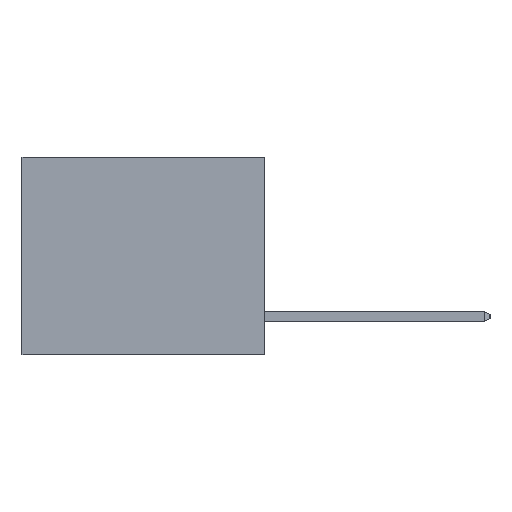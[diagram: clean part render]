
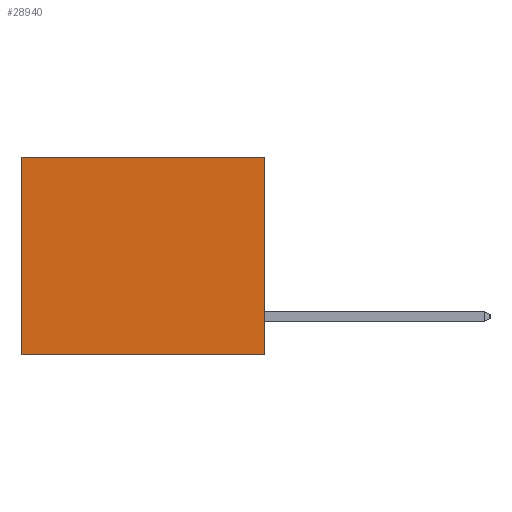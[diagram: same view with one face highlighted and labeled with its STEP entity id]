
A CAD part, left-side view. The second image highlights one B-rep face of the part: STEP entity #28940.
In plain terms, the highlighted planar face has unit normal (-1, 0, 0).
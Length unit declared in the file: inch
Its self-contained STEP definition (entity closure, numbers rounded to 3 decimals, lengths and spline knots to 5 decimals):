
#353 = LINE ( 'NONE', #3762, #6042 ) ;
#700 = CARTESIAN_POINT ( 'NONE',  ( 0.3165, 0.6, -0.49 ) ) ;
#1202 = DIRECTION ( 'NONE',  ( 0., 0., -1. ) ) ;
#1867 = ORIENTED_EDGE ( 'NONE', *, *, #23128, .F. ) ;
#2184 = ORIENTED_EDGE ( 'NONE', *, *, #22772, .T. ) ;
#2728 = FACE_OUTER_BOUND ( 'NONE', #9004, .T. ) ;
#3020 = CARTESIAN_POINT ( 'NONE',  ( 0.3165, 0., 0. ) ) ;
#3762 = CARTESIAN_POINT ( 'NONE',  ( 0.3165, 0., -0.49 ) ) ;
#4281 = ORIENTED_EDGE ( 'NONE', *, *, #28519, .F. ) ;
#4548 = DIRECTION ( 'NONE',  ( 0., 0., -1. ) ) ;
#4894 = VERTEX_POINT ( 'NONE', #14917 ) ;
#6042 = VECTOR ( 'NONE', #8673, 39.37008 ) ;
#6092 = DIRECTION ( 'NONE',  ( 1., 0., 0. ) ) ;
#6292 = PLANE ( 'NONE',  #20958 ) ;
#6659 = ORIENTED_EDGE ( 'NONE', *, *, #17720, .T. ) ;
#7152 = LINE ( 'NONE', #3020, #21429 ) ;
#8673 = DIRECTION ( 'NONE',  ( 0., 1., 0. ) ) ;
#9004 = EDGE_LOOP ( 'NONE', ( #2184, #1867, #4281, #6659 ) ) ;
#14641 = CARTESIAN_POINT ( 'NONE',  ( 0.3165, 0.6, -0.49 ) ) ;
#14892 = CARTESIAN_POINT ( 'NONE',  ( 0.3165, 0.6, 0. ) ) ;
#14917 = CARTESIAN_POINT ( 'NONE',  ( 0.3165, 0., -0.49 ) ) ;
#14937 = DIRECTION ( 'NONE',  ( 0., 0., -1. ) ) ;
#15644 = CARTESIAN_POINT ( 'NONE',  ( 0.3165, 0., -0.49 ) ) ;
#16626 = LINE ( 'NONE', #700, #28630 ) ;
#17720 = EDGE_CURVE ( 'NONE', #30732, #18672, #7152, .T. ) ;
#18672 = VERTEX_POINT ( 'NONE', #14892 ) ;
#18874 = VECTOR ( 'NONE', #4548, 39.37008 ) ;
#19816 = DIRECTION ( 'NONE',  ( 0., 1., 0. ) ) ;
#20418 = CARTESIAN_POINT ( 'NONE',  ( 0.3165, 0., 0. ) ) ;
#20958 = AXIS2_PLACEMENT_3D ( 'NONE', #15644, #6092, #1202 ) ;
#21429 = VECTOR ( 'NONE', #19816, 39.37008 ) ;
#22772 = EDGE_CURVE ( 'NONE', #18672, #26134, #16626, .T. ) ;
#23128 = EDGE_CURVE ( 'NONE', #4894, #26134, #353, .T. ) ;
#26134 = VERTEX_POINT ( 'NONE', #14641 ) ;
#26203 = CARTESIAN_POINT ( 'NONE',  ( 0.3165, 0., -0.49 ) ) ;
#28519 = EDGE_CURVE ( 'NONE', #30732, #4894, #29029, .T. ) ;
#28630 = VECTOR ( 'NONE', #14937, 39.37008 ) ;
#28940 = ADVANCED_FACE ( 'NONE', ( #2728 ), #6292, .F. ) ;
#29029 = LINE ( 'NONE', #26203, #18874 ) ;
#30732 = VERTEX_POINT ( 'NONE', #20418 ) ;
